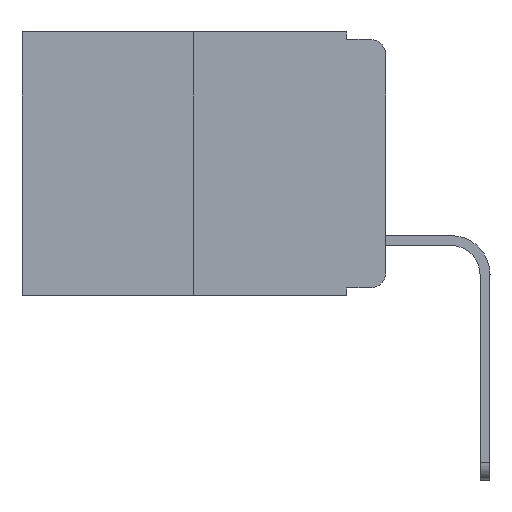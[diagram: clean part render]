
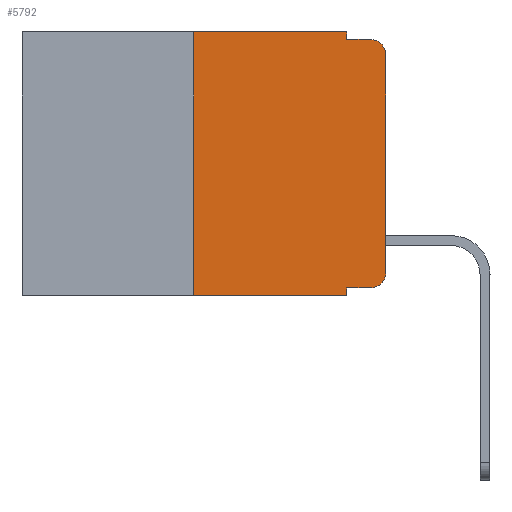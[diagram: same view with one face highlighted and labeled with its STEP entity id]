
A CAD part, left-side view. The second image highlights one B-rep face of the part: STEP entity #5792.
In plain terms, the highlighted planar face has unit normal (-1, 0, 0).
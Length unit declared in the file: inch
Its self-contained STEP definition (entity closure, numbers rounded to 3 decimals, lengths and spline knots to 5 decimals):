
#184 = DIRECTION ( 'NONE',  ( 0., 0., 1. ) ) ;
#213 = DIRECTION ( 'NONE',  ( 0., 0., -1. ) ) ;
#220 = VERTEX_POINT ( 'NONE', #3249 ) ;
#470 = EDGE_CURVE ( 'NONE', #9943, #1625, #5883, .T. ) ;
#637 = VECTOR ( 'NONE', #4108, 39.37008 ) ;
#787 = ORIENTED_EDGE ( 'NONE', *, *, #8984, .F. ) ;
#929 = CARTESIAN_POINT ( 'NONE',  ( 0., 0., -0.313 ) ) ;
#1075 = FACE_OUTER_BOUND ( 'NONE', #1431, .T. ) ;
#1176 = ORIENTED_EDGE ( 'NONE', *, *, #470, .F. ) ;
#1293 = LINE ( 'NONE', #3773, #3349 ) ;
#1324 = ORIENTED_EDGE ( 'NONE', *, *, #5298, .T. ) ;
#1431 = EDGE_LOOP ( 'NONE', ( #9121, #1324, #1176, #3102, #787, #8910, #9808, #8405, #2341, #3030 ) ) ;
#1559 = VERTEX_POINT ( 'NONE', #2644 ) ;
#1625 = VERTEX_POINT ( 'NONE', #3746 ) ;
#1856 = VECTOR ( 'NONE', #4661, 39.37008 ) ;
#1939 = AXIS2_PLACEMENT_3D ( 'NONE', #2620, #8583, #2662 ) ;
#2341 = ORIENTED_EDGE ( 'NONE', *, *, #9130, .T. ) ;
#2403 = EDGE_CURVE ( 'NONE', #6668, #7431, #4931, .T. ) ;
#2620 = CARTESIAN_POINT ( 'NONE',  ( 0., 0.473, 0. ) ) ;
#2644 = CARTESIAN_POINT ( 'NONE',  ( 0., 0.051, 0. ) ) ;
#2662 = DIRECTION ( 'NONE',  ( 0., 0., -1. ) ) ;
#2700 = CARTESIAN_POINT ( 'NONE',  ( 0., 0.02, -0.313 ) ) ;
#2818 = EDGE_CURVE ( 'NONE', #6369, #10800, #8058, .T. ) ;
#2859 = DIRECTION ( 'NONE',  ( 0., 0., -1. ) ) ;
#3030 = ORIENTED_EDGE ( 'NONE', *, *, #2818, .T. ) ;
#3102 = ORIENTED_EDGE ( 'NONE', *, *, #8473, .F. ) ;
#3137 = VERTEX_POINT ( 'NONE', #8109 ) ;
#3156 = VECTOR ( 'NONE', #7792, 39.37008 ) ;
#3170 = CARTESIAN_POINT ( 'NONE',  ( 0., 0.051, -0.01 ) ) ;
#3249 = CARTESIAN_POINT ( 'NONE',  ( 0., 0.25, 0. ) ) ;
#3347 = CARTESIAN_POINT ( 'NONE',  ( 0., 0.473, -0.343 ) ) ;
#3349 = VECTOR ( 'NONE', #5534, 39.37008 ) ;
#3562 = DIRECTION ( 'NONE',  ( 0., 0., 1. ) ) ;
#3623 = CARTESIAN_POINT ( 'NONE',  ( 0., 0.02, -0.03 ) ) ;
#3746 = CARTESIAN_POINT ( 'NONE',  ( 0., 0.02, -0.01 ) ) ;
#3773 = CARTESIAN_POINT ( 'NONE',  ( 0., 0.051, 0. ) ) ;
#4108 = DIRECTION ( 'NONE',  ( 0., -1., 0. ) ) ;
#4333 = VECTOR ( 'NONE', #3562, 39.37008 ) ;
#4338 = AXIS2_PLACEMENT_3D ( 'NONE', #3623, #4498, #213 ) ;
#4498 = DIRECTION ( 'NONE',  ( -1., 0., 0. ) ) ;
#4519 = LINE ( 'NONE', #6069, #3156 ) ;
#4661 = DIRECTION ( 'NONE',  ( 0., -1., 0. ) ) ;
#4744 = CARTESIAN_POINT ( 'NONE',  ( 0., 0.051, -0.333 ) ) ;
#4931 = LINE ( 'NONE', #10589, #7728 ) ;
#4993 = CARTESIAN_POINT ( 'NONE',  ( 0., 0.02, -0.333 ) ) ;
#5002 = VECTOR ( 'NONE', #184, 39.37008 ) ;
#5298 = EDGE_CURVE ( 'NONE', #9485, #1625, #10798, .T. ) ;
#5534 = DIRECTION ( 'NONE',  ( 0., 0., -1. ) ) ;
#5543 = CARTESIAN_POINT ( 'NONE',  ( 0., 0.051, -0.333 ) ) ;
#5685 = EDGE_CURVE ( 'NONE', #3137, #7431, #9447, .T. ) ;
#5792 = ADVANCED_FACE ( 'NONE', ( #1075 ), #9543, .F. ) ;
#5826 = CARTESIAN_POINT ( 'NONE',  ( 0., 0., 0. ) ) ;
#5883 = LINE ( 'NONE', #10062, #637 ) ;
#6069 = CARTESIAN_POINT ( 'NONE',  ( 0., 0.473, 0. ) ) ;
#6203 = CARTESIAN_POINT ( 'NONE',  ( 0., 0.25, 0. ) ) ;
#6369 = VERTEX_POINT ( 'NONE', #4993 ) ;
#6380 = EDGE_CURVE ( 'NONE', #10800, #9485, #6599, .T. ) ;
#6476 = EDGE_CURVE ( 'NONE', #3137, #220, #7524, .T. ) ;
#6599 = LINE ( 'NONE', #5826, #4333 ) ;
#6668 = VERTEX_POINT ( 'NONE', #5543 ) ;
#7431 = VERTEX_POINT ( 'NONE', #9345 ) ;
#7524 = LINE ( 'NONE', #6203, #5002 ) ;
#7544 = VECTOR ( 'NONE', #7638, 39.37008 ) ;
#7638 = DIRECTION ( 'NONE',  ( 0., -1., 0. ) ) ;
#7728 = VECTOR ( 'NONE', #2859, 39.37008 ) ;
#7792 = DIRECTION ( 'NONE',  ( 0., -1., 0. ) ) ;
#8058 = CIRCLE ( 'NONE', #9335, 0.02 ) ;
#8109 = CARTESIAN_POINT ( 'NONE',  ( 0., 0.25, -0.343 ) ) ;
#8405 = ORIENTED_EDGE ( 'NONE', *, *, #2403, .F. ) ;
#8473 = EDGE_CURVE ( 'NONE', #1559, #9943, #1293, .T. ) ;
#8583 = DIRECTION ( 'NONE',  ( 1., 0., 0. ) ) ;
#8679 = CARTESIAN_POINT ( 'NONE',  ( 0., 0., -0.03 ) ) ;
#8693 = DIRECTION ( 'NONE',  ( -1., 0., 0. ) ) ;
#8910 = ORIENTED_EDGE ( 'NONE', *, *, #6476, .F. ) ;
#8984 = EDGE_CURVE ( 'NONE', #220, #1559, #4519, .T. ) ;
#9121 = ORIENTED_EDGE ( 'NONE', *, *, #6380, .T. ) ;
#9130 = EDGE_CURVE ( 'NONE', #6668, #6369, #9674, .T. ) ;
#9335 = AXIS2_PLACEMENT_3D ( 'NONE', #2700, #8693, #9575 ) ;
#9345 = CARTESIAN_POINT ( 'NONE',  ( 0., 0.051, -0.343 ) ) ;
#9447 = LINE ( 'NONE', #3347, #7544 ) ;
#9485 = VERTEX_POINT ( 'NONE', #8679 ) ;
#9543 = PLANE ( 'NONE',  #1939 ) ;
#9575 = DIRECTION ( 'NONE',  ( 0., 0., -1. ) ) ;
#9674 = LINE ( 'NONE', #4744, #1856 ) ;
#9808 = ORIENTED_EDGE ( 'NONE', *, *, #5685, .T. ) ;
#9943 = VERTEX_POINT ( 'NONE', #3170 ) ;
#10062 = CARTESIAN_POINT ( 'NONE',  ( 0., 0.051, -0.01 ) ) ;
#10589 = CARTESIAN_POINT ( 'NONE',  ( 0., 0.051, 0. ) ) ;
#10798 = CIRCLE ( 'NONE', #4338, 0.02 ) ;
#10800 = VERTEX_POINT ( 'NONE', #929 ) ;
